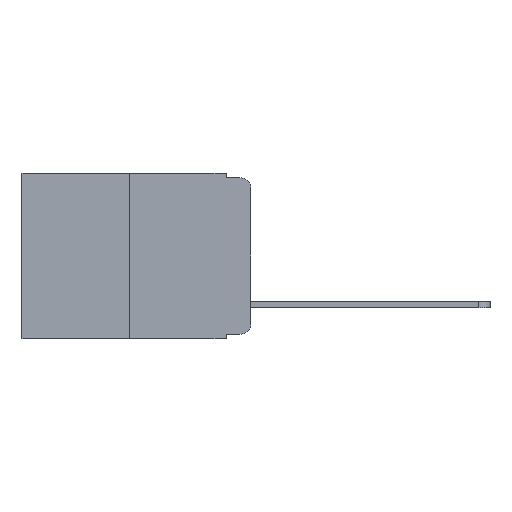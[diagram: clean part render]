
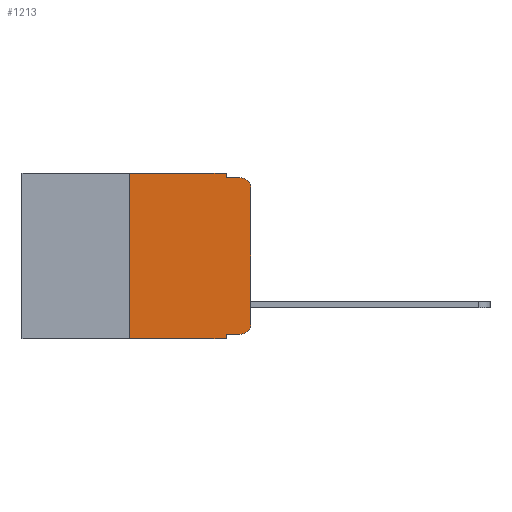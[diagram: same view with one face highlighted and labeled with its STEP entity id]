
A CAD part, left-side view. The second image highlights one B-rep face of the part: STEP entity #1213.
In plain terms, the highlighted planar face has unit normal (-1, 0, 0).
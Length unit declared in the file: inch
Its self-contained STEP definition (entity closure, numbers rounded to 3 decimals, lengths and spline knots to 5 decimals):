
#450 = AXIS2_PLACEMENT_3D ( 'NONE', #7569, #9356, #13006 ) ;
#624 = VERTEX_POINT ( 'NONE', #12873 ) ;
#700 = CIRCLE ( 'NONE', #3793, 0.02 ) ;
#727 = CARTESIAN_POINT ( 'NONE',  ( 0., 0.25, 0. ) ) ;
#941 = CARTESIAN_POINT ( 'NONE',  ( 0., 0.051, -0.01 ) ) ;
#1213 = ADVANCED_FACE ( 'NONE', ( #2787 ), #7264, .F. ) ;
#2787 = FACE_OUTER_BOUND ( 'NONE', #19633, .T. ) ;
#2905 = VERTEX_POINT ( 'NONE', #15255 ) ;
#2910 = LINE ( 'NONE', #16479, #10586 ) ;
#3172 = ORIENTED_EDGE ( 'NONE', *, *, #4597, .F. ) ;
#3625 = DIRECTION ( 'NONE',  ( 0., 0., -1. ) ) ;
#3680 = EDGE_CURVE ( 'NONE', #624, #20835, #2910, .T. ) ;
#3793 = AXIS2_PLACEMENT_3D ( 'NONE', #5252, #21638, #3625 ) ;
#3857 = VERTEX_POINT ( 'NONE', #22211 ) ;
#4274 = DIRECTION ( 'NONE',  ( 0., 0., 1. ) ) ;
#4332 = ORIENTED_EDGE ( 'NONE', *, *, #6070, .T. ) ;
#4424 = EDGE_CURVE ( 'NONE', #12799, #15666, #8019, .T. ) ;
#4597 = EDGE_CURVE ( 'NONE', #5622, #14971, #16779, .T. ) ;
#4622 = DIRECTION ( 'NONE',  ( 0., -1., 0. ) ) ;
#5066 = ORIENTED_EDGE ( 'NONE', *, *, #8630, .F. ) ;
#5154 = DIRECTION ( 'NONE',  ( 0., 0., -1. ) ) ;
#5252 = CARTESIAN_POINT ( 'NONE',  ( 0., 0.02, -0.03 ) ) ;
#5548 = EDGE_CURVE ( 'NONE', #2905, #12799, #19323, .T. ) ;
#5622 = VERTEX_POINT ( 'NONE', #6707 ) ;
#6070 = EDGE_CURVE ( 'NONE', #6094, #14971, #700, .T. ) ;
#6077 = VERTEX_POINT ( 'NONE', #19719 ) ;
#6094 = VERTEX_POINT ( 'NONE', #18121 ) ;
#6229 = CARTESIAN_POINT ( 'NONE',  ( 0., 0.051, -0.333 ) ) ;
#6349 = DIRECTION ( 'NONE',  ( 0., 0., 1. ) ) ;
#6486 = LINE ( 'NONE', #15262, #23435 ) ;
#6548 = CARTESIAN_POINT ( 'NONE',  ( 0., 0.02, -0.333 ) ) ;
#6707 = CARTESIAN_POINT ( 'NONE',  ( 0., 0.051, -0.01 ) ) ;
#6764 = LINE ( 'NONE', #13570, #17787 ) ;
#7264 = PLANE ( 'NONE',  #450 ) ;
#7410 = ORIENTED_EDGE ( 'NONE', *, *, #11989, .F. ) ;
#7485 = VECTOR ( 'NONE', #6349, 39.37008 ) ;
#7565 = ORIENTED_EDGE ( 'NONE', *, *, #15120, .F. ) ;
#7569 = CARTESIAN_POINT ( 'NONE',  ( 0., 0.473, 0. ) ) ;
#8019 = CIRCLE ( 'NONE', #19238, 0.02 ) ;
#8056 = LINE ( 'NONE', #727, #17102 ) ;
#8630 = EDGE_CURVE ( 'NONE', #624, #6077, #8056, .T. ) ;
#9103 = CARTESIAN_POINT ( 'NONE',  ( 0., 0.02, -0.01 ) ) ;
#9356 = DIRECTION ( 'NONE',  ( 1., 0., 0. ) ) ;
#9788 = DIRECTION ( 'NONE',  ( 0., -1., 0. ) ) ;
#10586 = VECTOR ( 'NONE', #18292, 39.37008 ) ;
#11199 = DIRECTION ( 'NONE',  ( -1., 0., 0. ) ) ;
#11578 = EDGE_CURVE ( 'NONE', #2905, #20835, #6486, .T. ) ;
#11688 = DIRECTION ( 'NONE',  ( 0., 0., -1. ) ) ;
#11800 = CARTESIAN_POINT ( 'NONE',  ( 0., 0., 0. ) ) ;
#11989 = EDGE_CURVE ( 'NONE', #3857, #5622, #6764, .T. ) ;
#12472 = ORIENTED_EDGE ( 'NONE', *, *, #11578, .F. ) ;
#12799 = VERTEX_POINT ( 'NONE', #6548 ) ;
#12873 = CARTESIAN_POINT ( 'NONE',  ( 0., 0.25, -0.343 ) ) ;
#13006 = DIRECTION ( 'NONE',  ( 0., 0., -1. ) ) ;
#13301 = ORIENTED_EDGE ( 'NONE', *, *, #4424, .T. ) ;
#13508 = VECTOR ( 'NONE', #9788, 39.37008 ) ;
#13570 = CARTESIAN_POINT ( 'NONE',  ( 0., 0.051, 0. ) ) ;
#13818 = CARTESIAN_POINT ( 'NONE',  ( 0., 0., -0.313 ) ) ;
#14971 = VERTEX_POINT ( 'NONE', #9103 ) ;
#15120 = EDGE_CURVE ( 'NONE', #6077, #3857, #17195, .T. ) ;
#15255 = CARTESIAN_POINT ( 'NONE',  ( 0., 0.051, -0.333 ) ) ;
#15262 = CARTESIAN_POINT ( 'NONE',  ( 0., 0.051, 0. ) ) ;
#15666 = VERTEX_POINT ( 'NONE', #13818 ) ;
#16479 = CARTESIAN_POINT ( 'NONE',  ( 0., 0.473, -0.343 ) ) ;
#16716 = ORIENTED_EDGE ( 'NONE', *, *, #19986, .T. ) ;
#16779 = LINE ( 'NONE', #941, #19347 ) ;
#17102 = VECTOR ( 'NONE', #4274, 39.37008 ) ;
#17195 = LINE ( 'NONE', #20625, #13508 ) ;
#17787 = VECTOR ( 'NONE', #5154, 39.37008 ) ;
#18121 = CARTESIAN_POINT ( 'NONE',  ( 0., 0., -0.03 ) ) ;
#18292 = DIRECTION ( 'NONE',  ( 0., -1., 0. ) ) ;
#18402 = ORIENTED_EDGE ( 'NONE', *, *, #3680, .T. ) ;
#18818 = CARTESIAN_POINT ( 'NONE',  ( 0., 0.02, -0.313 ) ) ;
#18971 = DIRECTION ( 'NONE',  ( 0., -1., 0. ) ) ;
#19238 = AXIS2_PLACEMENT_3D ( 'NONE', #18818, #11199, #22096 ) ;
#19323 = LINE ( 'NONE', #6229, #22703 ) ;
#19347 = VECTOR ( 'NONE', #18971, 39.37008 ) ;
#19633 = EDGE_LOOP ( 'NONE', ( #16716, #4332, #3172, #7410, #7565, #5066, #18402, #12472, #20806, #13301 ) ) ;
#19719 = CARTESIAN_POINT ( 'NONE',  ( 0., 0.25, 0. ) ) ;
#19986 = EDGE_CURVE ( 'NONE', #15666, #6094, #23325, .T. ) ;
#20625 = CARTESIAN_POINT ( 'NONE',  ( 0., 0.473, 0. ) ) ;
#20806 = ORIENTED_EDGE ( 'NONE', *, *, #5548, .T. ) ;
#20835 = VERTEX_POINT ( 'NONE', #21521 ) ;
#21521 = CARTESIAN_POINT ( 'NONE',  ( 0., 0.051, -0.343 ) ) ;
#21638 = DIRECTION ( 'NONE',  ( -1., 0., 0. ) ) ;
#22096 = DIRECTION ( 'NONE',  ( 0., 0., -1. ) ) ;
#22211 = CARTESIAN_POINT ( 'NONE',  ( 0., 0.051, 0. ) ) ;
#22703 = VECTOR ( 'NONE', #4622, 39.37008 ) ;
#23325 = LINE ( 'NONE', #11800, #7485 ) ;
#23435 = VECTOR ( 'NONE', #11688, 39.37008 ) ;
